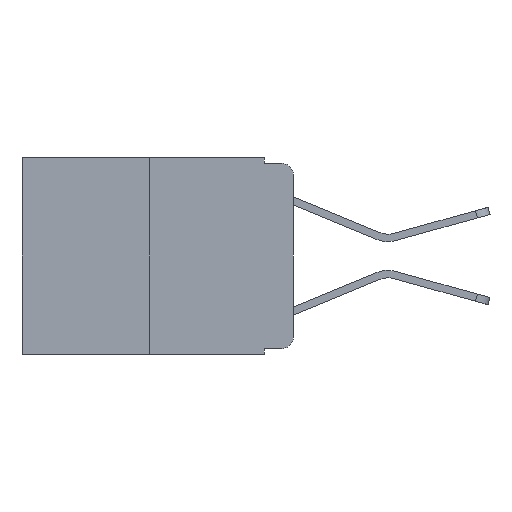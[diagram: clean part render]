
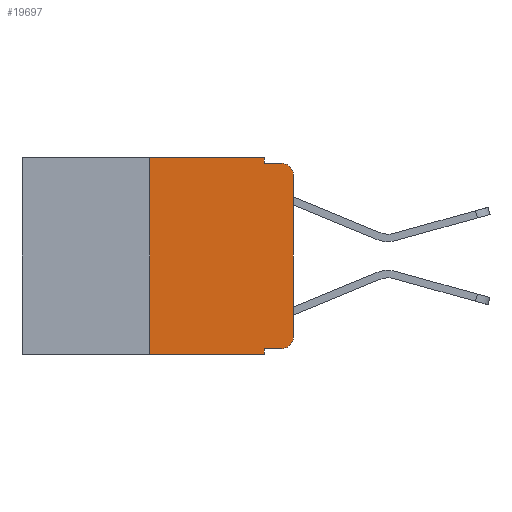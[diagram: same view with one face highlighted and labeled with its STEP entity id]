
A CAD part, left-side view. The second image highlights one B-rep face of the part: STEP entity #19697.
In plain terms, the highlighted planar face has unit normal (-1, 0, 0).
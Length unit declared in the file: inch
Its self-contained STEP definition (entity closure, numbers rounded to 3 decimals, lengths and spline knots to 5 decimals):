
#216 = DIRECTION ( 'NONE',  ( 0., 0., -1. ) ) ;
#226 = VERTEX_POINT ( 'NONE', #16225 ) ;
#238 = CARTESIAN_POINT ( 'NONE',  ( 0., 0.473, -0.343 ) ) ;
#335 = PLANE ( 'NONE',  #7310 ) ;
#645 = CARTESIAN_POINT ( 'NONE',  ( 0., 0.051, -0.01 ) ) ;
#1557 = DIRECTION ( 'NONE',  ( 0., 0., -1. ) ) ;
#1888 = EDGE_CURVE ( 'NONE', #2375, #15825, #13564, .T. ) ;
#2363 = VECTOR ( 'NONE', #20566, 39.37008 ) ;
#2375 = VERTEX_POINT ( 'NONE', #21376 ) ;
#2388 = VECTOR ( 'NONE', #10035, 39.37008 ) ;
#2638 = CARTESIAN_POINT ( 'NONE',  ( 0., 0., -0.03 ) ) ;
#3051 = DIRECTION ( 'NONE',  ( -1., 0., 0. ) ) ;
#3527 = VECTOR ( 'NONE', #19661, 39.37008 ) ;
#3878 = DIRECTION ( 'NONE',  ( 0., -1., 0. ) ) ;
#4419 = VERTEX_POINT ( 'NONE', #4991 ) ;
#4827 = EDGE_CURVE ( 'NONE', #16434, #7742, #18570, .T. ) ;
#4930 = VECTOR ( 'NONE', #17703, 39.37008 ) ;
#4991 = CARTESIAN_POINT ( 'NONE',  ( 0., 0.02, -0.333 ) ) ;
#4994 = CARTESIAN_POINT ( 'NONE',  ( 0., 0., 0. ) ) ;
#6287 = CARTESIAN_POINT ( 'NONE',  ( 0., 0., -0.313 ) ) ;
#6407 = VERTEX_POINT ( 'NONE', #2638 ) ;
#7076 = AXIS2_PLACEMENT_3D ( 'NONE', #17538, #3051, #12180 ) ;
#7310 = AXIS2_PLACEMENT_3D ( 'NONE', #11394, #15085, #22636 ) ;
#7742 = VERTEX_POINT ( 'NONE', #15350 ) ;
#7785 = VECTOR ( 'NONE', #3878, 39.37008 ) ;
#9341 = ORIENTED_EDGE ( 'NONE', *, *, #22909, .T. ) ;
#9368 = ORIENTED_EDGE ( 'NONE', *, *, #23188, .F. ) ;
#9507 = CARTESIAN_POINT ( 'NONE',  ( 0., 0.051, -0.333 ) ) ;
#9606 = EDGE_CURVE ( 'NONE', #18821, #23388, #13532, .T. ) ;
#9744 = VERTEX_POINT ( 'NONE', #6287 ) ;
#10035 = DIRECTION ( 'NONE',  ( 0., 0., 1. ) ) ;
#10548 = VECTOR ( 'NONE', #14151, 39.37008 ) ;
#10555 = EDGE_LOOP ( 'NONE', ( #21820, #12883, #12539, #9368, #22542, #21731, #9341, #16800, #17424, #14330 ) ) ;
#10591 = CARTESIAN_POINT ( 'NONE',  ( 0., 0.02, -0.01 ) ) ;
#10655 = DIRECTION ( 'NONE',  ( -1., 0., 0. ) ) ;
#11394 = CARTESIAN_POINT ( 'NONE',  ( 0., 0.473, 0. ) ) ;
#11631 = CARTESIAN_POINT ( 'NONE',  ( 0., 0.25, 0. ) ) ;
#11937 = EDGE_CURVE ( 'NONE', #4419, #9744, #19761, .T. ) ;
#12131 = EDGE_CURVE ( 'NONE', #6407, #23388, #22599, .T. ) ;
#12180 = DIRECTION ( 'NONE',  ( 0., 0., -1. ) ) ;
#12453 = CARTESIAN_POINT ( 'NONE',  ( 0., 0.051, 0. ) ) ;
#12539 = ORIENTED_EDGE ( 'NONE', *, *, #9606, .F. ) ;
#12883 = ORIENTED_EDGE ( 'NONE', *, *, #12131, .T. ) ;
#13168 = EDGE_CURVE ( 'NONE', #2375, #4419, #23132, .T. ) ;
#13532 = LINE ( 'NONE', #645, #2363 ) ;
#13564 = LINE ( 'NONE', #12453, #14422 ) ;
#14151 = DIRECTION ( 'NONE',  ( 0., -1., 0. ) ) ;
#14181 = CARTESIAN_POINT ( 'NONE',  ( 0., 0.02, -0.03 ) ) ;
#14330 = ORIENTED_EDGE ( 'NONE', *, *, #11937, .T. ) ;
#14422 = VECTOR ( 'NONE', #216, 39.37008 ) ;
#14581 = AXIS2_PLACEMENT_3D ( 'NONE', #14181, #10655, #1557 ) ;
#15085 = DIRECTION ( 'NONE',  ( 1., 0., 0. ) ) ;
#15152 = CARTESIAN_POINT ( 'NONE',  ( 0., 0.051, -0.01 ) ) ;
#15230 = EDGE_CURVE ( 'NONE', #226, #16434, #19874, .T. ) ;
#15350 = CARTESIAN_POINT ( 'NONE',  ( 0., 0.051, 0. ) ) ;
#15825 = VERTEX_POINT ( 'NONE', #16847 ) ;
#16059 = CARTESIAN_POINT ( 'NONE',  ( 0., 0.473, 0. ) ) ;
#16225 = CARTESIAN_POINT ( 'NONE',  ( 0., 0.25, -0.343 ) ) ;
#16434 = VERTEX_POINT ( 'NONE', #16605 ) ;
#16605 = CARTESIAN_POINT ( 'NONE',  ( 0., 0.25, 0. ) ) ;
#16800 = ORIENTED_EDGE ( 'NONE', *, *, #1888, .F. ) ;
#16847 = CARTESIAN_POINT ( 'NONE',  ( 0., 0.051, -0.343 ) ) ;
#17424 = ORIENTED_EDGE ( 'NONE', *, *, #13168, .T. ) ;
#17534 = LINE ( 'NONE', #238, #7785 ) ;
#17538 = CARTESIAN_POINT ( 'NONE',  ( 0., 0.02, -0.313 ) ) ;
#17703 = DIRECTION ( 'NONE',  ( 0., 0., -1. ) ) ;
#18103 = EDGE_CURVE ( 'NONE', #9744, #6407, #18707, .T. ) ;
#18570 = LINE ( 'NONE', #16059, #10548 ) ;
#18707 = LINE ( 'NONE', #4994, #3527 ) ;
#18801 = VECTOR ( 'NONE', #22369, 39.37008 ) ;
#18821 = VERTEX_POINT ( 'NONE', #15152 ) ;
#19661 = DIRECTION ( 'NONE',  ( 0., 0., 1. ) ) ;
#19697 = ADVANCED_FACE ( 'NONE', ( #20067 ), #335, .F. ) ;
#19761 = CIRCLE ( 'NONE', #7076, 0.02 ) ;
#19874 = LINE ( 'NONE', #11631, #2388 ) ;
#20067 = FACE_OUTER_BOUND ( 'NONE', #10555, .T. ) ;
#20566 = DIRECTION ( 'NONE',  ( 0., -1., 0. ) ) ;
#21376 = CARTESIAN_POINT ( 'NONE',  ( 0., 0.051, -0.333 ) ) ;
#21731 = ORIENTED_EDGE ( 'NONE', *, *, #15230, .F. ) ;
#21820 = ORIENTED_EDGE ( 'NONE', *, *, #18103, .T. ) ;
#21868 = LINE ( 'NONE', #22789, #4930 ) ;
#22369 = DIRECTION ( 'NONE',  ( 0., -1., 0. ) ) ;
#22542 = ORIENTED_EDGE ( 'NONE', *, *, #4827, .F. ) ;
#22599 = CIRCLE ( 'NONE', #14581, 0.02 ) ;
#22636 = DIRECTION ( 'NONE',  ( 0., 0., -1. ) ) ;
#22789 = CARTESIAN_POINT ( 'NONE',  ( 0., 0.051, 0. ) ) ;
#22909 = EDGE_CURVE ( 'NONE', #226, #15825, #17534, .T. ) ;
#23132 = LINE ( 'NONE', #9507, #18801 ) ;
#23188 = EDGE_CURVE ( 'NONE', #7742, #18821, #21868, .T. ) ;
#23388 = VERTEX_POINT ( 'NONE', #10591 ) ;
